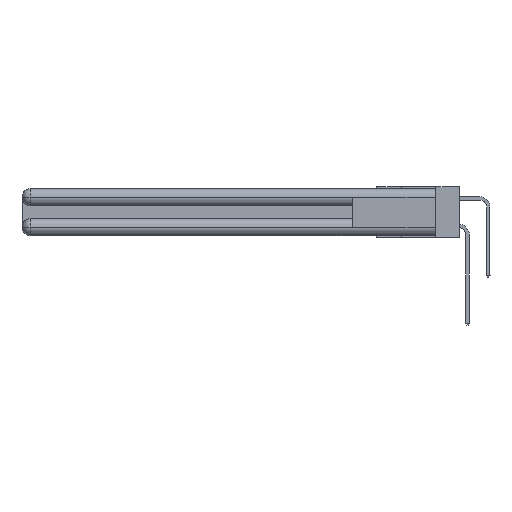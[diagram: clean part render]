
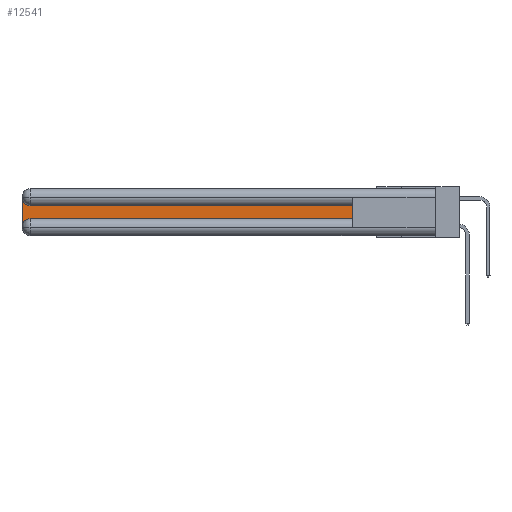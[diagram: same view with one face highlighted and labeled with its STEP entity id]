
A CAD part, left-side view. The second image highlights one B-rep face of the part: STEP entity #12541.
In plain terms, the highlighted planar face has unit normal (-1, 0, 0).
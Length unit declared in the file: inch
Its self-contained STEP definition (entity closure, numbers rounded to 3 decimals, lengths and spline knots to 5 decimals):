
#188 = ORIENTED_EDGE ( 'NONE', *, *, #6189, .T. ) ;
#1027 = ORIENTED_EDGE ( 'NONE', *, *, #28854, .T. ) ;
#4753 = DIRECTION ( 'NONE',  ( 1., 0., 0. ) ) ;
#4882 = CARTESIAN_POINT ( 'NONE',  ( 0.075, 2.94, -0.0625 ) ) ;
#4996 = AXIS2_PLACEMENT_3D ( 'NONE', #37577, #20111, #25973 ) ;
#6189 = EDGE_CURVE ( 'NONE', #36188, #36030, #16103, .T. ) ;
#6898 = ORIENTED_EDGE ( 'NONE', *, *, #30400, .T. ) ;
#8800 = LINE ( 'NONE', #26466, #31218 ) ;
#8957 = DIRECTION ( 'NONE',  ( 0., 1., 0. ) ) ;
#9333 = CARTESIAN_POINT ( 'NONE',  ( 0.075, 0.6, -0.2175 ) ) ;
#9573 = DIRECTION ( 'NONE',  ( 1., 0., 0. ) ) ;
#9750 = CARTESIAN_POINT ( 'NONE',  ( 0.075, 0.6, -0.2175 ) ) ;
#9923 = EDGE_CURVE ( 'NONE', #36305, #36188, #31421, .T. ) ;
#11036 = EDGE_CURVE ( 'NONE', #35199, #27507, #16197, .T. ) ;
#12541 = ADVANCED_FACE ( 'NONE', ( #15691 ), #28676, .F. ) ;
#15196 = VECTOR ( 'NONE', #35741, 39.37008 ) ;
#15691 = FACE_OUTER_BOUND ( 'NONE', #22322, .T. ) ;
#15700 = AXIS2_PLACEMENT_3D ( 'NONE', #23878, #9573, #35999 ) ;
#16103 = LINE ( 'NONE', #21255, #35731 ) ;
#16197 = CIRCLE ( 'NONE', #25276, 0.06 ) ;
#18362 = CARTESIAN_POINT ( 'NONE',  ( 0.075, 2.94, -0.1225 ) ) ;
#19451 = CARTESIAN_POINT ( 'NONE',  ( 0.075, 3., -0.2175 ) ) ;
#20111 = DIRECTION ( 'NONE',  ( 1., 0., 0. ) ) ;
#20651 = EDGE_CURVE ( 'NONE', #27655, #35199, #8800, .T. ) ;
#21255 = CARTESIAN_POINT ( 'NONE',  ( 0.075, 0.6, -0.2175 ) ) ;
#21313 = CARTESIAN_POINT ( 'NONE',  ( 0.075, 3., -0.0625 ) ) ;
#22322 = EDGE_LOOP ( 'NONE', ( #34549, #27093, #1027, #36435, #188, #6898 ) ) ;
#23106 = VECTOR ( 'NONE', #33517, 39.37008 ) ;
#23878 = CARTESIAN_POINT ( 'NONE',  ( 0.075, 2.94, -0.2775 ) ) ;
#25276 = AXIS2_PLACEMENT_3D ( 'NONE', #4882, #4753, #28626 ) ;
#25973 = DIRECTION ( 'NONE',  ( 0., 0., -1. ) ) ;
#26466 = CARTESIAN_POINT ( 'NONE',  ( 0.075, 0.6, -0.1225 ) ) ;
#27093 = ORIENTED_EDGE ( 'NONE', *, *, #11036, .T. ) ;
#27507 = VERTEX_POINT ( 'NONE', #21313 ) ;
#27655 = VERTEX_POINT ( 'NONE', #28196 ) ;
#28196 = CARTESIAN_POINT ( 'NONE',  ( 0.075, 0.6, -0.1225 ) ) ;
#28626 = DIRECTION ( 'NONE',  ( 0., 0., -1. ) ) ;
#28676 = PLANE ( 'NONE',  #4996 ) ;
#28854 = EDGE_CURVE ( 'NONE', #27507, #36305, #29066, .T. ) ;
#29066 = LINE ( 'NONE', #19451, #23106 ) ;
#30400 = EDGE_CURVE ( 'NONE', #36030, #27655, #31685, .T. ) ;
#31218 = VECTOR ( 'NONE', #8957, 39.37008 ) ;
#31421 = CIRCLE ( 'NONE', #15700, 0.06 ) ;
#31685 = LINE ( 'NONE', #9333, #15196 ) ;
#32895 = DIRECTION ( 'NONE',  ( 0., -1., 0. ) ) ;
#33517 = DIRECTION ( 'NONE',  ( 0., 0., -1. ) ) ;
#34549 = ORIENTED_EDGE ( 'NONE', *, *, #20651, .T. ) ;
#35199 = VERTEX_POINT ( 'NONE', #18362 ) ;
#35731 = VECTOR ( 'NONE', #32895, 39.37008 ) ;
#35741 = DIRECTION ( 'NONE',  ( 0., 0., 1. ) ) ;
#35999 = DIRECTION ( 'NONE',  ( 0., 0., -1. ) ) ;
#36030 = VERTEX_POINT ( 'NONE', #9750 ) ;
#36188 = VERTEX_POINT ( 'NONE', #37057 ) ;
#36305 = VERTEX_POINT ( 'NONE', #37571 ) ;
#36435 = ORIENTED_EDGE ( 'NONE', *, *, #9923, .T. ) ;
#37057 = CARTESIAN_POINT ( 'NONE',  ( 0.075, 2.94, -0.2175 ) ) ;
#37571 = CARTESIAN_POINT ( 'NONE',  ( 0.075, 3., -0.2775 ) ) ;
#37577 = CARTESIAN_POINT ( 'NONE',  ( 0.075, 3., -0.1225 ) ) ;
